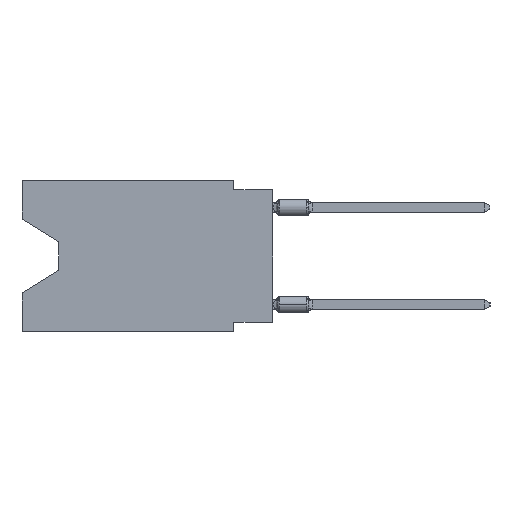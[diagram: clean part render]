
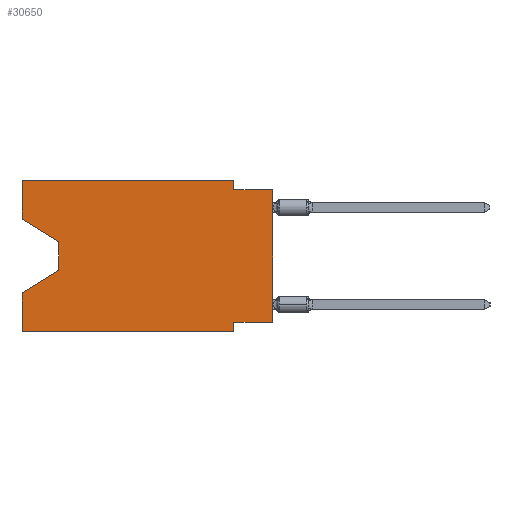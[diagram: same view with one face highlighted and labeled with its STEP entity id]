
A CAD part, left-side view. The second image highlights one B-rep face of the part: STEP entity #30650.
In plain terms, the highlighted planar face has unit normal (-1, 0, 0).
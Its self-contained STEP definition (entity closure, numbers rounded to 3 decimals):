
#11 = EDGE_CURVE ( 'NONE', #29043, #3822, #24539, .T. ) ;
#354 = CARTESIAN_POINT ( 'NONE',  ( 0., 16.383, 0. ) ) ;
#602 = VERTEX_POINT ( 'NONE', #3755 ) ;
#714 = CARTESIAN_POINT ( 'NONE',  ( 0., 0., -9.271 ) ) ;
#857 = DIRECTION ( 'NONE',  ( 0., -1., 0. ) ) ;
#1419 = EDGE_CURVE ( 'NONE', #4877, #22641, #15997, .T. ) ;
#2055 = VECTOR ( 'NONE', #25680, 1000. ) ;
#2124 = CARTESIAN_POINT ( 'NONE',  ( 0., 2.54, 0. ) ) ;
#2566 = DIRECTION ( 'NONE',  ( 0., 0., -1. ) ) ;
#2893 = CARTESIAN_POINT ( 'NONE',  ( 0., 16.383, 0. ) ) ;
#3739 = LINE ( 'NONE', #25219, #23182 ) ;
#3755 = CARTESIAN_POINT ( 'NONE',  ( 0., 16.383, -9.906 ) ) ;
#3796 = CARTESIAN_POINT ( 'NONE',  ( 0., 2.54, -9.906 ) ) ;
#3822 = VERTEX_POINT ( 'NONE', #17102 ) ;
#4172 = LINE ( 'NONE', #30702, #13356 ) ;
#4672 = EDGE_CURVE ( 'NONE', #30707, #10100, #4859, .T. ) ;
#4859 = LINE ( 'NONE', #14978, #31208 ) ;
#4877 = VERTEX_POINT ( 'NONE', #15433 ) ;
#5778 = VECTOR ( 'NONE', #24863, 1000. ) ;
#6164 = EDGE_CURVE ( 'NONE', #3822, #4877, #3739, .T. ) ;
#6196 = LINE ( 'NONE', #29903, #9928 ) ;
#6310 = EDGE_CURVE ( 'NONE', #29043, #18429, #26312, .T. ) ;
#6474 = LINE ( 'NONE', #27969, #7015 ) ;
#6700 = DIRECTION ( 'NONE',  ( 0., 0., -1. ) ) ;
#7015 = VECTOR ( 'NONE', #18017, 1000. ) ;
#8184 = CARTESIAN_POINT ( 'NONE',  ( 0., 2.54, 0. ) ) ;
#8330 = ORIENTED_EDGE ( 'NONE', *, *, #11091, .F. ) ;
#8438 = EDGE_CURVE ( 'NONE', #602, #22641, #24518, .T. ) ;
#9027 = CARTESIAN_POINT ( 'NONE',  ( 0., 13.97, -5.893 ) ) ;
#9037 = EDGE_CURVE ( 'NONE', #18429, #22300, #26193, .T. ) ;
#9408 = ORIENTED_EDGE ( 'NONE', *, *, #6310, .F. ) ;
#9928 = VECTOR ( 'NONE', #857, 1000. ) ;
#10100 = VERTEX_POINT ( 'NONE', #10581 ) ;
#10581 = CARTESIAN_POINT ( 'NONE',  ( 0., 0., -0.635 ) ) ;
#10597 = CARTESIAN_POINT ( 'NONE',  ( 0., 16.383, -2.546 ) ) ;
#11091 = EDGE_CURVE ( 'NONE', #26073, #13437, #4172, .T. ) ;
#11356 = ORIENTED_EDGE ( 'NONE', *, *, #8438, .F. ) ;
#11473 = VECTOR ( 'NONE', #28150, 1000. ) ;
#11827 = ORIENTED_EDGE ( 'NONE', *, *, #11, .T. ) ;
#12244 = DIRECTION ( 'NONE',  ( 0., 1., 0. ) ) ;
#12530 = DIRECTION ( 'NONE',  ( 0., 0., 1. ) ) ;
#12580 = ORIENTED_EDGE ( 'NONE', *, *, #9037, .F. ) ;
#13356 = VECTOR ( 'NONE', #26434, 1000. ) ;
#13437 = VERTEX_POINT ( 'NONE', #3796 ) ;
#14348 = CARTESIAN_POINT ( 'NONE',  ( 0., 16.383, 0. ) ) ;
#14496 = DIRECTION ( 'NONE',  ( 0., -1., 0. ) ) ;
#14689 = ORIENTED_EDGE ( 'NONE', *, *, #16615, .F. ) ;
#14978 = CARTESIAN_POINT ( 'NONE',  ( 0., 0., -0.635 ) ) ;
#15433 = CARTESIAN_POINT ( 'NONE',  ( 0., 13.97, -5.893 ) ) ;
#15580 = EDGE_CURVE ( 'NONE', #602, #13437, #6196, .T. ) ;
#15997 = LINE ( 'NONE', #9027, #11473 ) ;
#16464 = ORIENTED_EDGE ( 'NONE', *, *, #1419, .T. ) ;
#16615 = EDGE_CURVE ( 'NONE', #22300, #30707, #16967, .T. ) ;
#16967 = LINE ( 'NONE', #2124, #29681 ) ;
#17102 = CARTESIAN_POINT ( 'NONE',  ( 0., 13.97, -4.013 ) ) ;
#17818 = VECTOR ( 'NONE', #12244, 1000. ) ;
#17948 = ORIENTED_EDGE ( 'NONE', *, *, #23084, .F. ) ;
#18017 = DIRECTION ( 'NONE',  ( 0., 0., 1. ) ) ;
#18429 = VERTEX_POINT ( 'NONE', #354 ) ;
#18533 = EDGE_CURVE ( 'NONE', #30037, #10100, #6474, .T. ) ;
#18720 = VECTOR ( 'NONE', #28877, 1000. ) ;
#19449 = PLANE ( 'NONE',  #28996 ) ;
#19950 = CARTESIAN_POINT ( 'NONE',  ( 0., 16.383, -2.546 ) ) ;
#20087 = EDGE_LOOP ( 'NONE', ( #11827, #27346, #16464, #11356, #29180, #8330, #17948, #23496, #25676, #14689, #12580, #9408 ) ) ;
#20774 = CARTESIAN_POINT ( 'NONE',  ( 0., 0., -9.271 ) ) ;
#21556 = CARTESIAN_POINT ( 'NONE',  ( 0., 2.54, -9.271 ) ) ;
#21659 = DIRECTION ( 'NONE',  ( 1., 0., 0. ) ) ;
#22300 = VERTEX_POINT ( 'NONE', #8184 ) ;
#22327 = LINE ( 'NONE', #714, #17818 ) ;
#22641 = VERTEX_POINT ( 'NONE', #24421 ) ;
#23084 = EDGE_CURVE ( 'NONE', #30037, #26073, #22327, .T. ) ;
#23182 = VECTOR ( 'NONE', #28053, 1000. ) ;
#23496 = ORIENTED_EDGE ( 'NONE', *, *, #18533, .T. ) ;
#24421 = CARTESIAN_POINT ( 'NONE',  ( 0., 16.383, -7.36 ) ) ;
#24518 = LINE ( 'NONE', #2893, #28859 ) ;
#24539 = LINE ( 'NONE', #19950, #5778 ) ;
#24863 = DIRECTION ( 'NONE',  ( 0., -0.855, -0.519 ) ) ;
#25219 = CARTESIAN_POINT ( 'NONE',  ( 0., 13.97, -4.013 ) ) ;
#25676 = ORIENTED_EDGE ( 'NONE', *, *, #4672, .F. ) ;
#25680 = DIRECTION ( 'NONE',  ( 0., 0., 1. ) ) ;
#26073 = VERTEX_POINT ( 'NONE', #21556 ) ;
#26193 = LINE ( 'NONE', #14348, #18720 ) ;
#26312 = LINE ( 'NONE', #28842, #2055 ) ;
#26434 = DIRECTION ( 'NONE',  ( 0., 0., -1. ) ) ;
#26727 = CARTESIAN_POINT ( 'NONE',  ( 0., 2.54, -0.635 ) ) ;
#27346 = ORIENTED_EDGE ( 'NONE', *, *, #6164, .T. ) ;
#27969 = CARTESIAN_POINT ( 'NONE',  ( 0., 0., 0. ) ) ;
#28053 = DIRECTION ( 'NONE',  ( 0., 0., -1. ) ) ;
#28150 = DIRECTION ( 'NONE',  ( 0., 0.855, -0.519 ) ) ;
#28842 = CARTESIAN_POINT ( 'NONE',  ( 0., 16.383, 0. ) ) ;
#28859 = VECTOR ( 'NONE', #12530, 1000. ) ;
#28877 = DIRECTION ( 'NONE',  ( 0., -1., 0. ) ) ;
#28996 = AXIS2_PLACEMENT_3D ( 'NONE', #29262, #21659, #2566 ) ;
#29043 = VERTEX_POINT ( 'NONE', #10597 ) ;
#29097 = FACE_OUTER_BOUND ( 'NONE', #20087, .T. ) ;
#29180 = ORIENTED_EDGE ( 'NONE', *, *, #15580, .T. ) ;
#29262 = CARTESIAN_POINT ( 'NONE',  ( 0., 16.383, 0. ) ) ;
#29681 = VECTOR ( 'NONE', #6700, 1000. ) ;
#29903 = CARTESIAN_POINT ( 'NONE',  ( 0., 16.383, -9.906 ) ) ;
#30037 = VERTEX_POINT ( 'NONE', #20774 ) ;
#30650 = ADVANCED_FACE ( 'NONE', ( #29097 ), #19449, .F. ) ;
#30702 = CARTESIAN_POINT ( 'NONE',  ( 0., 2.54, -9.906 ) ) ;
#30707 = VERTEX_POINT ( 'NONE', #26727 ) ;
#31208 = VECTOR ( 'NONE', #14496, 1000. ) ;
